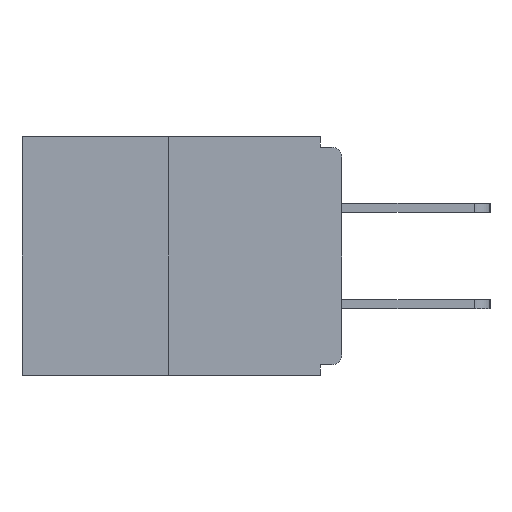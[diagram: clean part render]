
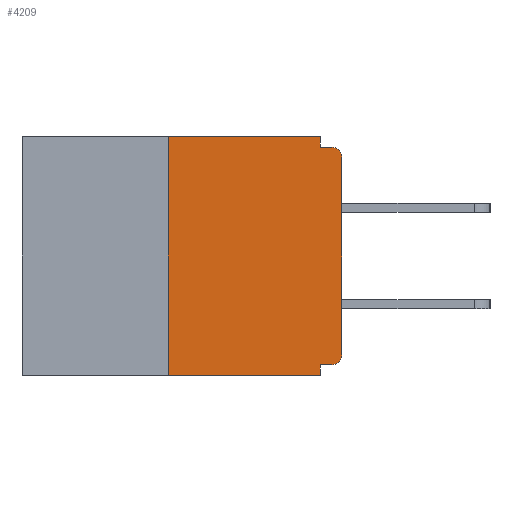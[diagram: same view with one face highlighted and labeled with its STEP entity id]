
A CAD part, left-side view. The second image highlights one B-rep face of the part: STEP entity #4209.
In plain terms, the highlighted planar face has unit normal (-1, 0, 0).
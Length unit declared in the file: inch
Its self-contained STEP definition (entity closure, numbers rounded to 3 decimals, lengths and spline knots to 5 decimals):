
#244 = CARTESIAN_POINT ( 'NONE',  ( 0., 0.46, -0.343 ) ) ;
#517 = CARTESIAN_POINT ( 'NONE',  ( 0., 0.015, -0.328 ) ) ;
#701 = DIRECTION ( 'NONE',  ( -1., 0., 0. ) ) ;
#756 = ORIENTED_EDGE ( 'NONE', *, *, #23713, .F. ) ;
#771 = VECTOR ( 'NONE', #5728, 39.37008 ) ;
#998 = CARTESIAN_POINT ( 'NONE',  ( 0., 0.031, -0.328 ) ) ;
#1079 = DIRECTION ( 'NONE',  ( 0., 0., -1. ) ) ;
#1297 = DIRECTION ( 'NONE',  ( 0., 0., -1. ) ) ;
#2025 = ORIENTED_EDGE ( 'NONE', *, *, #10773, .T. ) ;
#2602 = EDGE_LOOP ( 'NONE', ( #18062, #19931, #2025, #6341, #6015, #5905, #5932, #14035, #3930, #756 ) ) ;
#2803 = LINE ( 'NONE', #16426, #18807 ) ;
#2867 = CARTESIAN_POINT ( 'NONE',  ( 0., 0.031, -0.343 ) ) ;
#3189 = VERTEX_POINT ( 'NONE', #22838 ) ;
#3930 = ORIENTED_EDGE ( 'NONE', *, *, #18829, .F. ) ;
#3949 = DIRECTION ( 'NONE',  ( 0., -1., 0. ) ) ;
#3981 = DIRECTION ( 'NONE',  ( 0., 0., -1. ) ) ;
#4048 = DIRECTION ( 'NONE',  ( 0., -1., 0. ) ) ;
#4209 = ADVANCED_FACE ( 'NONE', ( #8729 ), #9561, .F. ) ;
#5200 = VECTOR ( 'NONE', #1297, 39.37008 ) ;
#5474 = AXIS2_PLACEMENT_3D ( 'NONE', #15907, #23775, #1079 ) ;
#5580 = VECTOR ( 'NONE', #19647, 39.37008 ) ;
#5728 = DIRECTION ( 'NONE',  ( 0., 0., 1. ) ) ;
#5905 = ORIENTED_EDGE ( 'NONE', *, *, #7856, .T. ) ;
#5924 = DIRECTION ( 'NONE',  ( 0., 0., -1. ) ) ;
#5932 = ORIENTED_EDGE ( 'NONE', *, *, #18922, .T. ) ;
#6015 = ORIENTED_EDGE ( 'NONE', *, *, #19259, .F. ) ;
#6039 = CARTESIAN_POINT ( 'NONE',  ( 0., 0., -0.328 ) ) ;
#6341 = ORIENTED_EDGE ( 'NONE', *, *, #10200, .F. ) ;
#6469 = CARTESIAN_POINT ( 'NONE',  ( 0., 0., 0. ) ) ;
#6489 = LINE ( 'NONE', #19175, #23869 ) ;
#6536 = AXIS2_PLACEMENT_3D ( 'NONE', #15151, #22721, #5924 ) ;
#6696 = CARTESIAN_POINT ( 'NONE',  ( 0., 0.031, -0.343 ) ) ;
#7189 = CARTESIAN_POINT ( 'NONE',  ( 0., 0., -0.03 ) ) ;
#7467 = CARTESIAN_POINT ( 'NONE',  ( 0., 0.015, -0.015 ) ) ;
#7608 = LINE ( 'NONE', #9385, #23215 ) ;
#7856 = EDGE_CURVE ( 'NONE', #21929, #14466, #18308, .T. ) ;
#8531 = VERTEX_POINT ( 'NONE', #2867 ) ;
#8729 = FACE_OUTER_BOUND ( 'NONE', #2602, .T. ) ;
#8742 = LINE ( 'NONE', #244, #9935 ) ;
#8803 = AXIS2_PLACEMENT_3D ( 'NONE', #19851, #701, #14021 ) ;
#9385 = CARTESIAN_POINT ( 'NONE',  ( 0., 0.031, 0. ) ) ;
#9561 = PLANE ( 'NONE',  #6536 ) ;
#9935 = VECTOR ( 'NONE', #3949, 39.37008 ) ;
#10174 = VERTEX_POINT ( 'NONE', #18006 ) ;
#10200 = EDGE_CURVE ( 'NONE', #22107, #8531, #15232, .T. ) ;
#10773 = EDGE_CURVE ( 'NONE', #3189, #8531, #8742, .T. ) ;
#11217 = VERTEX_POINT ( 'NONE', #7189 ) ;
#11422 = CARTESIAN_POINT ( 'NONE',  ( 0., 0.25, 0. ) ) ;
#11507 = VECTOR ( 'NONE', #15266, 39.37008 ) ;
#11815 = LINE ( 'NONE', #6039, #11507 ) ;
#14021 = DIRECTION ( 'NONE',  ( 0., 0., -1. ) ) ;
#14035 = ORIENTED_EDGE ( 'NONE', *, *, #22062, .T. ) ;
#14466 = VERTEX_POINT ( 'NONE', #14697 ) ;
#14697 = CARTESIAN_POINT ( 'NONE',  ( 0., 0., -0.313 ) ) ;
#15151 = CARTESIAN_POINT ( 'NONE',  ( 0., 0.46, 0. ) ) ;
#15232 = LINE ( 'NONE', #6696, #5200 ) ;
#15266 = DIRECTION ( 'NONE',  ( 0., 1., 0. ) ) ;
#15330 = LINE ( 'NONE', #6469, #5580 ) ;
#15907 = CARTESIAN_POINT ( 'NONE',  ( 0., 0.015, -0.03 ) ) ;
#15960 = CARTESIAN_POINT ( 'NONE',  ( 0., 0.031, 0. ) ) ;
#16426 = CARTESIAN_POINT ( 'NONE',  ( 0., 0.46, 0. ) ) ;
#17154 = CARTESIAN_POINT ( 'NONE',  ( 0., 0.25, 0. ) ) ;
#17629 = VERTEX_POINT ( 'NONE', #17154 ) ;
#18006 = CARTESIAN_POINT ( 'NONE',  ( 0., 0.031, -0.015 ) ) ;
#18062 = ORIENTED_EDGE ( 'NONE', *, *, #24426, .F. ) ;
#18235 = LINE ( 'NONE', #11422, #771 ) ;
#18308 = CIRCLE ( 'NONE', #8803, 0.015 ) ;
#18807 = VECTOR ( 'NONE', #22167, 39.37008 ) ;
#18829 = EDGE_CURVE ( 'NONE', #10174, #22448, #6489, .T. ) ;
#18922 = EDGE_CURVE ( 'NONE', #14466, #11217, #15330, .T. ) ;
#19175 = CARTESIAN_POINT ( 'NONE',  ( 0., 0., -0.015 ) ) ;
#19259 = EDGE_CURVE ( 'NONE', #21929, #22107, #11815, .T. ) ;
#19647 = DIRECTION ( 'NONE',  ( 0., 0., 1. ) ) ;
#19851 = CARTESIAN_POINT ( 'NONE',  ( 0., 0.015, -0.313 ) ) ;
#19931 = ORIENTED_EDGE ( 'NONE', *, *, #20578, .F. ) ;
#20578 = EDGE_CURVE ( 'NONE', #3189, #17629, #18235, .T. ) ;
#21929 = VERTEX_POINT ( 'NONE', #517 ) ;
#22062 = EDGE_CURVE ( 'NONE', #11217, #22448, #23740, .T. ) ;
#22107 = VERTEX_POINT ( 'NONE', #998 ) ;
#22167 = DIRECTION ( 'NONE',  ( 0., -1., 0. ) ) ;
#22448 = VERTEX_POINT ( 'NONE', #7467 ) ;
#22614 = VERTEX_POINT ( 'NONE', #15960 ) ;
#22721 = DIRECTION ( 'NONE',  ( 1., 0., 0. ) ) ;
#22838 = CARTESIAN_POINT ( 'NONE',  ( 0., 0.25, -0.343 ) ) ;
#23215 = VECTOR ( 'NONE', #3981, 39.37008 ) ;
#23713 = EDGE_CURVE ( 'NONE', #22614, #10174, #7608, .T. ) ;
#23740 = CIRCLE ( 'NONE', #5474, 0.015 ) ;
#23775 = DIRECTION ( 'NONE',  ( -1., 0., 0. ) ) ;
#23869 = VECTOR ( 'NONE', #4048, 39.37008 ) ;
#24426 = EDGE_CURVE ( 'NONE', #17629, #22614, #2803, .T. ) ;
